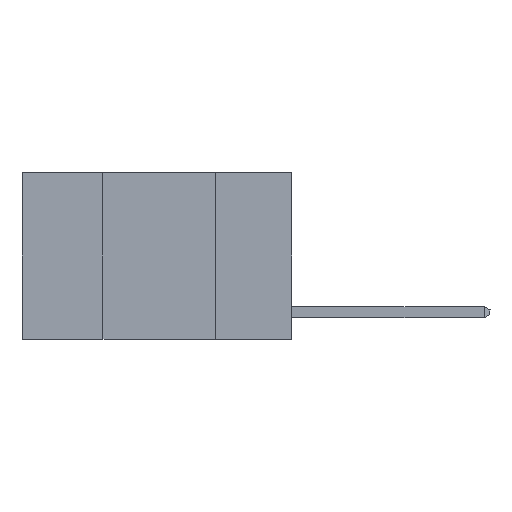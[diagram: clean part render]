
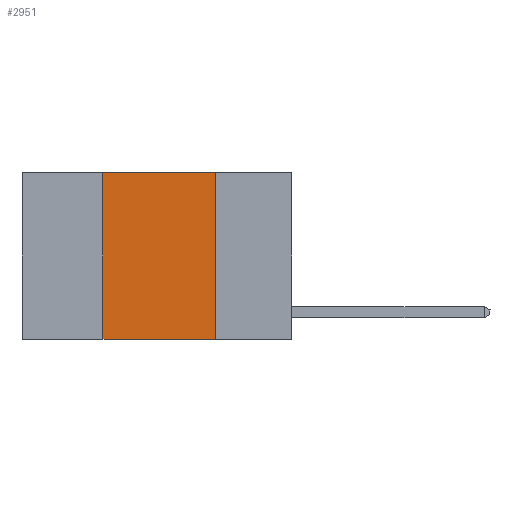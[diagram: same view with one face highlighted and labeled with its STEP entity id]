
A CAD part, left-side view. The second image highlights one B-rep face of the part: STEP entity #2951.
In plain terms, the highlighted planar face has unit normal (-1, 0, 0).
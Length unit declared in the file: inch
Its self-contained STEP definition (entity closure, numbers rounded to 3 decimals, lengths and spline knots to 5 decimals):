
#275 = VECTOR ( 'NONE', #4035, 39.37008 ) ;
#353 = VERTEX_POINT ( 'NONE', #19743 ) ;
#461 = ORIENTED_EDGE ( 'NONE', *, *, #18747, .F. ) ;
#538 = VERTEX_POINT ( 'NONE', #27372 ) ;
#912 = EDGE_LOOP ( 'NONE', ( #4854, #461, #25285, #30323 ) ) ;
#1460 = LINE ( 'NONE', #2227, #5511 ) ;
#2227 = CARTESIAN_POINT ( 'NONE',  ( 0., 0.42, 0. ) ) ;
#2951 = ADVANCED_FACE ( 'NONE', ( #14281 ), #19567, .F. ) ;
#3138 = DIRECTION ( 'NONE',  ( 1., 0., 0. ) ) ;
#4035 = DIRECTION ( 'NONE',  ( 0., 0., -1. ) ) ;
#4854 = ORIENTED_EDGE ( 'NONE', *, *, #19739, .F. ) ;
#5511 = VECTOR ( 'NONE', #23532, 39.37008 ) ;
#5819 = LINE ( 'NONE', #22834, #275 ) ;
#6655 = VERTEX_POINT ( 'NONE', #6987 ) ;
#6987 = CARTESIAN_POINT ( 'NONE',  ( 0., 0.17, -0.37 ) ) ;
#7797 = VECTOR ( 'NONE', #16396, 39.37008 ) ;
#7818 = DIRECTION ( 'NONE',  ( 0., 0., -1. ) ) ;
#7998 = EDGE_CURVE ( 'NONE', #538, #353, #1460, .T. ) ;
#9656 = LINE ( 'NONE', #30022, #7797 ) ;
#14281 = FACE_OUTER_BOUND ( 'NONE', #912, .T. ) ;
#14492 = CARTESIAN_POINT ( 'NONE',  ( 0., 0.6, 0. ) ) ;
#14596 = VECTOR ( 'NONE', #29415, 39.37008 ) ;
#16396 = DIRECTION ( 'NONE',  ( 0., -1., 0. ) ) ;
#17495 = LINE ( 'NONE', #29615, #14596 ) ;
#18747 = EDGE_CURVE ( 'NONE', #353, #26446, #17495, .T. ) ;
#19567 = PLANE ( 'NONE',  #29795 ) ;
#19739 = EDGE_CURVE ( 'NONE', #26446, #6655, #5819, .T. ) ;
#19743 = CARTESIAN_POINT ( 'NONE',  ( 0., 0.42, 0. ) ) ;
#22834 = CARTESIAN_POINT ( 'NONE',  ( 0., 0.17, 0. ) ) ;
#23405 = EDGE_CURVE ( 'NONE', #538, #6655, #9656, .T. ) ;
#23532 = DIRECTION ( 'NONE',  ( 0., 0., 1. ) ) ;
#25285 = ORIENTED_EDGE ( 'NONE', *, *, #7998, .F. ) ;
#26355 = CARTESIAN_POINT ( 'NONE',  ( 0., 0.17, 0. ) ) ;
#26446 = VERTEX_POINT ( 'NONE', #26355 ) ;
#27372 = CARTESIAN_POINT ( 'NONE',  ( 0., 0.42, -0.37 ) ) ;
#29415 = DIRECTION ( 'NONE',  ( 0., -1., 0. ) ) ;
#29615 = CARTESIAN_POINT ( 'NONE',  ( 0., 0.6, 0. ) ) ;
#29795 = AXIS2_PLACEMENT_3D ( 'NONE', #14492, #3138, #7818 ) ;
#30022 = CARTESIAN_POINT ( 'NONE',  ( 0., 0.6, -0.37 ) ) ;
#30323 = ORIENTED_EDGE ( 'NONE', *, *, #23405, .T. ) ;
